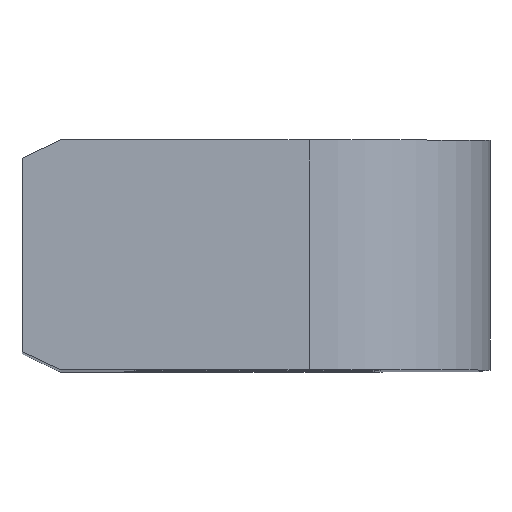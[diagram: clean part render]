
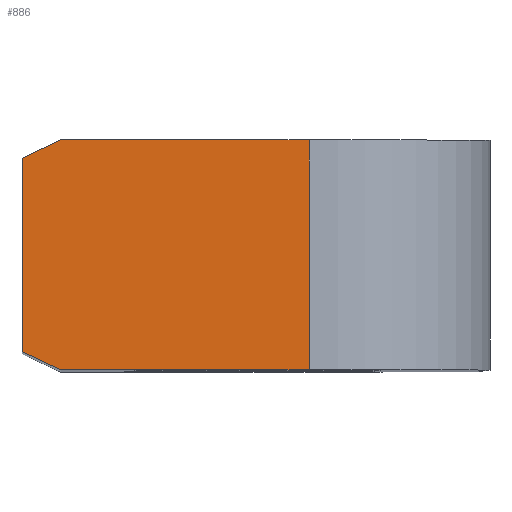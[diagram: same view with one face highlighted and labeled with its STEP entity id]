
A CAD part, top view. The second image highlights one B-rep face of the part: STEP entity #886.
In plain terms, the highlighted planar face has unit normal (0, 0, 1).
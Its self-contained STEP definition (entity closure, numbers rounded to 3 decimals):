
#20 = VERTEX_POINT ( 'NONE', #712 ) ;
#41 = CARTESIAN_POINT ( 'NONE',  ( 1.072, 6.35, 0. ) ) ;
#53 = CARTESIAN_POINT ( 'NONE',  ( 0., 6.35, 0. ) ) ;
#57 = ORIENTED_EDGE ( 'NONE', *, *, #1002, .T. ) ;
#75 = DIRECTION ( 'NONE',  ( 0., 1., 0. ) ) ;
#77 = ORIENTED_EDGE ( 'NONE', *, *, #175, .T. ) ;
#103 = CARTESIAN_POINT ( 'NONE',  ( 0., 0., 0. ) ) ;
#135 = VERTEX_POINT ( 'NONE', #894 ) ;
#143 = FACE_OUTER_BOUND ( 'NONE', #1052, .T. ) ;
#167 = VERTEX_POINT ( 'NONE', #988 ) ;
#175 = EDGE_CURVE ( 'NONE', #534, #135, #861, .T. ) ;
#186 = ORIENTED_EDGE ( 'NONE', *, *, #495, .F. ) ;
#201 = ORIENTED_EDGE ( 'NONE', *, *, #796, .T. ) ;
#270 = DIRECTION ( 'NONE',  ( 1., 0., 0. ) ) ;
#283 = CARTESIAN_POINT ( 'NONE',  ( 0., 0.5, 0. ) ) ;
#294 = VERTEX_POINT ( 'NONE', #523 ) ;
#363 = CARTESIAN_POINT ( 'NONE',  ( 7.929, 6.35, 0. ) ) ;
#389 = DIRECTION ( 'NONE',  ( 0., 0., -1. ) ) ;
#414 = CARTESIAN_POINT ( 'NONE',  ( 0., 6.35, 0. ) ) ;
#468 = VECTOR ( 'NONE', #697, 1000. ) ;
#492 = VERTEX_POINT ( 'NONE', #363 ) ;
#495 = EDGE_CURVE ( 'NONE', #294, #492, #885, .T. ) ;
#523 = CARTESIAN_POINT ( 'NONE',  ( 1.072, 6.35, 0. ) ) ;
#534 = VERTEX_POINT ( 'NONE', #694 ) ;
#559 = LINE ( 'NONE', #283, #740 ) ;
#576 = AXIS2_PLACEMENT_3D ( 'NONE', #53, #389, #977 ) ;
#595 = ORIENTED_EDGE ( 'NONE', *, *, #994, .T. ) ;
#611 = EDGE_CURVE ( 'NONE', #20, #534, #559, .T. ) ;
#634 = VECTOR ( 'NONE', #75, 1000. ) ;
#690 = CARTESIAN_POINT ( 'NONE',  ( 0., 6.35, 0. ) ) ;
#694 = CARTESIAN_POINT ( 'NONE',  ( 1.072, 0., 0. ) ) ;
#696 = DIRECTION ( 'NONE',  ( -0.906, -0.423, 0. ) ) ;
#697 = DIRECTION ( 'NONE',  ( 1., 0., 0. ) ) ;
#707 = VECTOR ( 'NONE', #270, 1000. ) ;
#712 = CARTESIAN_POINT ( 'NONE',  ( 0., 0.5, 0. ) ) ;
#718 = CARTESIAN_POINT ( 'NONE',  ( 7.929, 6.35, 0. ) ) ;
#740 = VECTOR ( 'NONE', #837, 1000. ) ;
#749 = VECTOR ( 'NONE', #696, 1000. ) ;
#796 = EDGE_CURVE ( 'NONE', #294, #167, #851, .T. ) ;
#811 = DIRECTION ( 'NONE',  ( 0., -1., 0. ) ) ;
#813 = LINE ( 'NONE', #414, #862 ) ;
#837 = DIRECTION ( 'NONE',  ( 0.906, -0.423, 0. ) ) ;
#851 = LINE ( 'NONE', #41, #749 ) ;
#861 = LINE ( 'NONE', #103, #707 ) ;
#862 = VECTOR ( 'NONE', #811, 1000. ) ;
#885 = LINE ( 'NONE', #690, #468 ) ;
#886 = ADVANCED_FACE ( 'NONE', ( #143 ), #965, .F. ) ;
#894 = CARTESIAN_POINT ( 'NONE',  ( 7.929, 0., 0. ) ) ;
#934 = ORIENTED_EDGE ( 'NONE', *, *, #611, .T. ) ;
#965 = PLANE ( 'NONE',  #576 ) ;
#977 = DIRECTION ( 'NONE',  ( -1., 0., 0. ) ) ;
#988 = CARTESIAN_POINT ( 'NONE',  ( 0., 5.85, 0. ) ) ;
#994 = EDGE_CURVE ( 'NONE', #167, #20, #813, .T. ) ;
#1002 = EDGE_CURVE ( 'NONE', #135, #492, #1024, .T. ) ;
#1024 = LINE ( 'NONE', #718, #634 ) ;
#1052 = EDGE_LOOP ( 'NONE', ( #595, #934, #77, #57, #186, #201 ) ) ;
